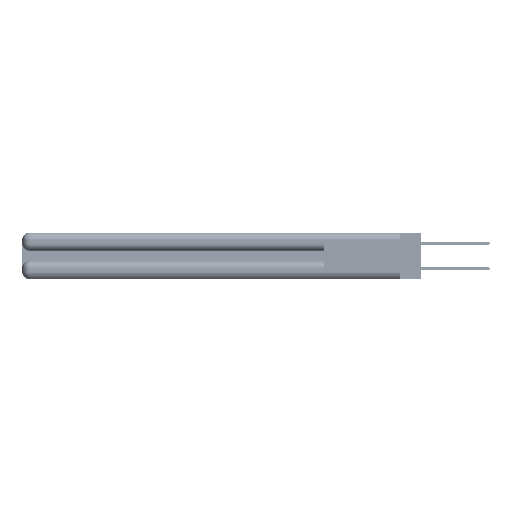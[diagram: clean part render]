
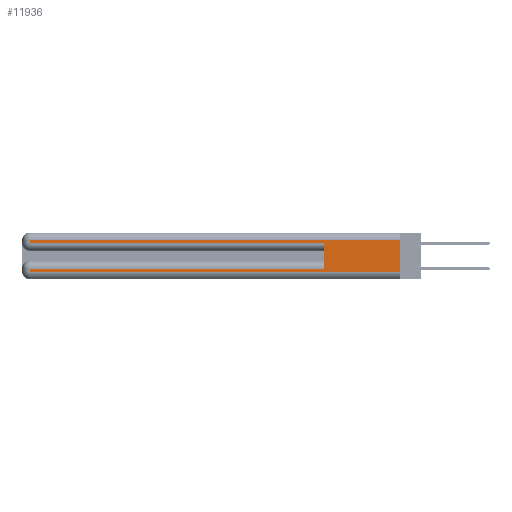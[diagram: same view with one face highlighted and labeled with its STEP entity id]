
A CAD part, left-side view. The second image highlights one B-rep face of the part: STEP entity #11936.
In plain terms, the highlighted planar face has unit normal (-1, 0, 0).
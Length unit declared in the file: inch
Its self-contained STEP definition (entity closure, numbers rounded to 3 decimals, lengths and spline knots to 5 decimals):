
#2 = ORIENTED_EDGE ( 'NONE', *, *, #2137, .T. ) ;
#1174 = CARTESIAN_POINT ( 'NONE',  ( 0., 2.94, 0.37 ) ) ;
#1587 = ORIENTED_EDGE ( 'NONE', *, *, #49072, .T. ) ;
#2137 = EDGE_CURVE ( 'NONE', #9208, #28840, #30361, .T. ) ;
#2308 = CARTESIAN_POINT ( 'NONE',  ( 0., 2.94, 0.37 ) ) ;
#2927 = PLANE ( 'NONE',  #46827 ) ;
#3815 = VECTOR ( 'NONE', #38327, 39.37008 ) ;
#5031 = CARTESIAN_POINT ( 'NONE',  ( 0., 0., 0.085 ) ) ;
#5394 = DIRECTION ( 'NONE',  ( 0., 0., -1. ) ) ;
#7139 = DIRECTION ( 'NONE',  ( 0., 0., -1. ) ) ;
#7505 = EDGE_CURVE ( 'NONE', #22473, #24426, #25866, .T. ) ;
#7791 = LINE ( 'NONE', #42391, #38384 ) ;
#8214 = VECTOR ( 'NONE', #5394, 39.37008 ) ;
#8335 = LINE ( 'NONE', #23143, #40205 ) ;
#8829 = ORIENTED_EDGE ( 'NONE', *, *, #47265, .T. ) ;
#9169 = DIRECTION ( 'NONE',  ( 0., 0., -1. ) ) ;
#9208 = VERTEX_POINT ( 'NONE', #40507 ) ;
#9426 = ORIENTED_EDGE ( 'NONE', *, *, #32402, .T. ) ;
#9558 = LINE ( 'NONE', #2308, #19345 ) ;
#10240 = VECTOR ( 'NONE', #46904, 39.37008 ) ;
#10451 = VERTEX_POINT ( 'NONE', #48018 ) ;
#11936 = ADVANCED_FACE ( 'NONE', ( #53312 ), #2927, .F. ) ;
#13318 = ORIENTED_EDGE ( 'NONE', *, *, #32164, .F. ) ;
#15361 = ORIENTED_EDGE ( 'NONE', *, *, #29932, .T. ) ;
#17797 = LINE ( 'NONE', #44307, #27548 ) ;
#17856 = CARTESIAN_POINT ( 'NONE',  ( 0., 0.6, 0.145 ) ) ;
#19345 = VECTOR ( 'NONE', #39811, 39.37008 ) ;
#20014 = LINE ( 'NONE', #17856, #10240 ) ;
#21666 = DIRECTION ( 'NONE',  ( 0., 1., 0. ) ) ;
#22473 = VERTEX_POINT ( 'NONE', #32179 ) ;
#22577 = VERTEX_POINT ( 'NONE', #32707 ) ;
#23143 = CARTESIAN_POINT ( 'NONE',  ( 0., 0., 0.285 ) ) ;
#24426 = VERTEX_POINT ( 'NONE', #40710 ) ;
#25866 = LINE ( 'NONE', #38276, #38219 ) ;
#26110 = VERTEX_POINT ( 'NONE', #42894 ) ;
#27548 = VECTOR ( 'NONE', #48489, 39.37008 ) ;
#28840 = VERTEX_POINT ( 'NONE', #51441 ) ;
#29932 = EDGE_CURVE ( 'NONE', #28840, #22577, #8335, .T. ) ;
#30361 = LINE ( 'NONE', #1174, #8214 ) ;
#30429 = ORIENTED_EDGE ( 'NONE', *, *, #7505, .F. ) ;
#30900 = EDGE_CURVE ( 'NONE', #33722, #10451, #37064, .T. ) ;
#32073 = DIRECTION ( 'NONE',  ( 1., 0., 0. ) ) ;
#32164 = EDGE_CURVE ( 'NONE', #33722, #22577, #20014, .T. ) ;
#32179 = CARTESIAN_POINT ( 'NONE',  ( 0., 0., 0.31 ) ) ;
#32402 = EDGE_CURVE ( 'NONE', #10451, #26110, #9558, .T. ) ;
#32707 = CARTESIAN_POINT ( 'NONE',  ( 0., 0.6, 0.285 ) ) ;
#33722 = VERTEX_POINT ( 'NONE', #51467 ) ;
#37064 = LINE ( 'NONE', #5031, #3815 ) ;
#38219 = VECTOR ( 'NONE', #9169, 39.37008 ) ;
#38276 = CARTESIAN_POINT ( 'NONE',  ( 0., 0., 0.37 ) ) ;
#38327 = DIRECTION ( 'NONE',  ( 0., 1., 0. ) ) ;
#38384 = VECTOR ( 'NONE', #21666, 39.37008 ) ;
#39811 = DIRECTION ( 'NONE',  ( 0., 0., -1. ) ) ;
#40205 = VECTOR ( 'NONE', #52219, 39.37008 ) ;
#40507 = CARTESIAN_POINT ( 'NONE',  ( 0., 2.94, 0.31 ) ) ;
#40710 = CARTESIAN_POINT ( 'NONE',  ( 0., 0., 0.06 ) ) ;
#42391 = CARTESIAN_POINT ( 'NONE',  ( 0., 0., 0.31 ) ) ;
#42894 = CARTESIAN_POINT ( 'NONE',  ( 0., 2.94, 0.06 ) ) ;
#44307 = CARTESIAN_POINT ( 'NONE',  ( 0., 0., 0.06 ) ) ;
#44402 = CARTESIAN_POINT ( 'NONE',  ( 0., 0., 0.37 ) ) ;
#46827 = AXIS2_PLACEMENT_3D ( 'NONE', #44402, #32073, #7139 ) ;
#46904 = DIRECTION ( 'NONE',  ( 0., 0., 1. ) ) ;
#47265 = EDGE_CURVE ( 'NONE', #26110, #24426, #17797, .T. ) ;
#48018 = CARTESIAN_POINT ( 'NONE',  ( 0., 2.94, 0.085 ) ) ;
#48489 = DIRECTION ( 'NONE',  ( 0., -1., 0. ) ) ;
#49072 = EDGE_CURVE ( 'NONE', #22473, #9208, #7791, .T. ) ;
#50349 = ORIENTED_EDGE ( 'NONE', *, *, #30900, .T. ) ;
#50994 = EDGE_LOOP ( 'NONE', ( #30429, #1587, #2, #15361, #13318, #50349, #9426, #8829 ) ) ;
#51441 = CARTESIAN_POINT ( 'NONE',  ( 0., 2.94, 0.285 ) ) ;
#51467 = CARTESIAN_POINT ( 'NONE',  ( 0., 0.6, 0.085 ) ) ;
#52219 = DIRECTION ( 'NONE',  ( 0., -1., 0. ) ) ;
#53312 = FACE_OUTER_BOUND ( 'NONE', #50994, .T. ) ;
